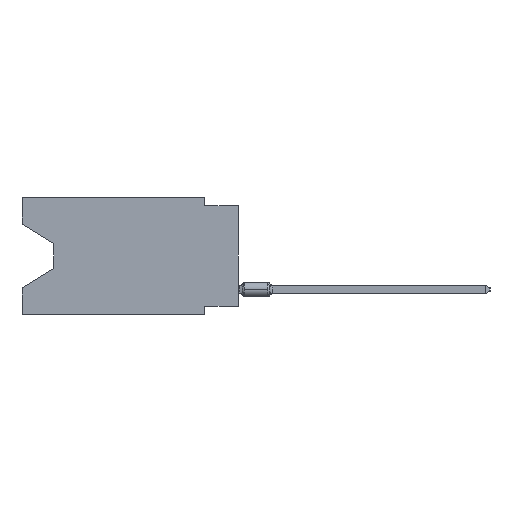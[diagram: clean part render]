
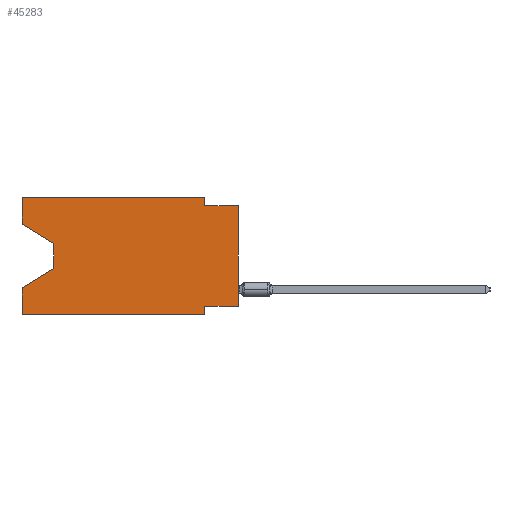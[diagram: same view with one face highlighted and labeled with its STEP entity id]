
A CAD part, left-side view. The second image highlights one B-rep face of the part: STEP entity #45283.
In plain terms, the highlighted planar face has unit normal (-1, 0, 0).
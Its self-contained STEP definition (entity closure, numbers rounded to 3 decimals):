
#516 = EDGE_CURVE ( 'NONE', #14917, #9543, #1992, .T. ) ;
#1327 = CARTESIAN_POINT ( 'NONE',  ( 0., 13.97, -5.385 ) ) ;
#1767 = LINE ( 'NONE', #17411, #11857 ) ;
#1992 = LINE ( 'NONE', #2253, #34191 ) ;
#2253 = CARTESIAN_POINT ( 'NONE',  ( 0., 16.383, -2.038 ) ) ;
#2542 = VECTOR ( 'NONE', #33363, 1000. ) ;
#2892 = VERTEX_POINT ( 'NONE', #22735 ) ;
#2940 = LINE ( 'NONE', #46184, #41017 ) ;
#3522 = CARTESIAN_POINT ( 'NONE',  ( 0., 16.383, 0. ) ) ;
#3793 = DIRECTION ( 'NONE',  ( 1., 0., 0. ) ) ;
#3966 = VECTOR ( 'NONE', #41997, 1000. ) ;
#4473 = VECTOR ( 'NONE', #34867, 1000. ) ;
#5000 = LINE ( 'NONE', #12959, #21048 ) ;
#5082 = CARTESIAN_POINT ( 'NONE',  ( 0., 16.383, 0. ) ) ;
#6580 = CARTESIAN_POINT ( 'NONE',  ( 0., 0., -8.255 ) ) ;
#6715 = LINE ( 'NONE', #37948, #2542 ) ;
#6970 = VECTOR ( 'NONE', #30922, 1000. ) ;
#7168 = ORIENTED_EDGE ( 'NONE', *, *, #42177, .F. ) ;
#8255 = VERTEX_POINT ( 'NONE', #30023 ) ;
#8639 = VERTEX_POINT ( 'NONE', #40820 ) ;
#9111 = DIRECTION ( 'NONE',  ( 0., -1., 0. ) ) ;
#9205 = EDGE_CURVE ( 'NONE', #42547, #8639, #19503, .T. ) ;
#9543 = VERTEX_POINT ( 'NONE', #41468 ) ;
#11857 = VECTOR ( 'NONE', #32268, 1000. ) ;
#12143 = EDGE_CURVE ( 'NONE', #8255, #49991, #5000, .T. ) ;
#12901 = CARTESIAN_POINT ( 'NONE',  ( 0., 0., 0. ) ) ;
#12959 = CARTESIAN_POINT ( 'NONE',  ( 0., 0., -0.635 ) ) ;
#13042 = ORIENTED_EDGE ( 'NONE', *, *, #18100, .F. ) ;
#14010 = EDGE_CURVE ( 'NONE', #20271, #48665, #39620, .T. ) ;
#14073 = CARTESIAN_POINT ( 'NONE',  ( 0., 16.383, -6.852 ) ) ;
#14858 = CARTESIAN_POINT ( 'NONE',  ( 0., 16.383, -8.89 ) ) ;
#14917 = VERTEX_POINT ( 'NONE', #18050 ) ;
#15325 = LINE ( 'NONE', #15568, #6970 ) ;
#15461 = EDGE_CURVE ( 'NONE', #22792, #8639, #39693, .T. ) ;
#15568 = CARTESIAN_POINT ( 'NONE',  ( 0., 13.97, -3.505 ) ) ;
#16507 = PLANE ( 'NONE',  #19033 ) ;
#16711 = CARTESIAN_POINT ( 'NONE',  ( 0., 16.383, 0. ) ) ;
#17411 = CARTESIAN_POINT ( 'NONE',  ( 0., 2.54, 0. ) ) ;
#18050 = CARTESIAN_POINT ( 'NONE',  ( 0., 16.383, -2.038 ) ) ;
#18100 = EDGE_CURVE ( 'NONE', #2892, #8255, #1767, .T. ) ;
#18133 = DIRECTION ( 'NONE',  ( 0., -0.855, -0.519 ) ) ;
#19033 = AXIS2_PLACEMENT_3D ( 'NONE', #3522, #3793, #38588 ) ;
#19503 = LINE ( 'NONE', #42770, #4473 ) ;
#20271 = VERTEX_POINT ( 'NONE', #1327 ) ;
#21048 = VECTOR ( 'NONE', #9111, 1000. ) ;
#21423 = ORIENTED_EDGE ( 'NONE', *, *, #14010, .T. ) ;
#22512 = CARTESIAN_POINT ( 'NONE',  ( 0., 0., -0.635 ) ) ;
#22615 = ORIENTED_EDGE ( 'NONE', *, *, #15461, .F. ) ;
#22735 = CARTESIAN_POINT ( 'NONE',  ( 0., 2.54, 0. ) ) ;
#22792 = VERTEX_POINT ( 'NONE', #42399 ) ;
#22929 = ORIENTED_EDGE ( 'NONE', *, *, #12143, .F. ) ;
#24029 = CARTESIAN_POINT ( 'NONE',  ( 0., 13.97, -5.385 ) ) ;
#24306 = LINE ( 'NONE', #5082, #40575 ) ;
#24942 = EDGE_CURVE ( 'NONE', #29100, #49991, #47685, .T. ) ;
#27446 = CARTESIAN_POINT ( 'NONE',  ( 0., 16.383, 0. ) ) ;
#27990 = DIRECTION ( 'NONE',  ( 0., 0., 1. ) ) ;
#28440 = DIRECTION ( 'NONE',  ( 0., 0., -1. ) ) ;
#29100 = VERTEX_POINT ( 'NONE', #6580 ) ;
#29361 = EDGE_LOOP ( 'NONE', ( #46754, #34235, #21423, #42304, #40164, #22615, #49719, #36845, #22929, #13042, #7168, #47385 ) ) ;
#30023 = CARTESIAN_POINT ( 'NONE',  ( 0., 2.54, -0.635 ) ) ;
#30922 = DIRECTION ( 'NONE',  ( 0., 0., -1. ) ) ;
#31504 = VECTOR ( 'NONE', #34871, 1000. ) ;
#32268 = DIRECTION ( 'NONE',  ( 0., 0., -1. ) ) ;
#33363 = DIRECTION ( 'NONE',  ( 0., 1., 0. ) ) ;
#33942 = EDGE_CURVE ( 'NONE', #29100, #22792, #6715, .T. ) ;
#34191 = VECTOR ( 'NONE', #18133, 1000. ) ;
#34235 = ORIENTED_EDGE ( 'NONE', *, *, #37583, .T. ) ;
#34695 = EDGE_CURVE ( 'NONE', #42547, #48665, #2940, .T. ) ;
#34867 = DIRECTION ( 'NONE',  ( 0., -1., 0. ) ) ;
#34871 = DIRECTION ( 'NONE',  ( 0., -1., 0. ) ) ;
#36845 = ORIENTED_EDGE ( 'NONE', *, *, #24942, .T. ) ;
#37583 = EDGE_CURVE ( 'NONE', #9543, #20271, #15325, .T. ) ;
#37948 = CARTESIAN_POINT ( 'NONE',  ( 0., 0., -8.255 ) ) ;
#38336 = FACE_OUTER_BOUND ( 'NONE', #29361, .T. ) ;
#38588 = DIRECTION ( 'NONE',  ( 0., 0., -1. ) ) ;
#39620 = LINE ( 'NONE', #24029, #3966 ) ;
#39693 = LINE ( 'NONE', #47622, #44975 ) ;
#39892 = DIRECTION ( 'NONE',  ( 0., 0., 1. ) ) ;
#40164 = ORIENTED_EDGE ( 'NONE', *, *, #9205, .T. ) ;
#40575 = VECTOR ( 'NONE', #39892, 1000. ) ;
#40820 = CARTESIAN_POINT ( 'NONE',  ( 0., 2.54, -8.89 ) ) ;
#41017 = VECTOR ( 'NONE', #49275, 1000. ) ;
#41468 = CARTESIAN_POINT ( 'NONE',  ( 0., 13.97, -3.505 ) ) ;
#41997 = DIRECTION ( 'NONE',  ( 0., 0.855, -0.519 ) ) ;
#42177 = EDGE_CURVE ( 'NONE', #49962, #2892, #42529, .T. ) ;
#42304 = ORIENTED_EDGE ( 'NONE', *, *, #34695, .F. ) ;
#42399 = CARTESIAN_POINT ( 'NONE',  ( 0., 2.54, -8.255 ) ) ;
#42529 = LINE ( 'NONE', #27446, #31504 ) ;
#42547 = VERTEX_POINT ( 'NONE', #14858 ) ;
#42733 = EDGE_CURVE ( 'NONE', #14917, #49962, #24306, .T. ) ;
#42770 = CARTESIAN_POINT ( 'NONE',  ( 0., 16.383, -8.89 ) ) ;
#44006 = VECTOR ( 'NONE', #27990, 1000. ) ;
#44975 = VECTOR ( 'NONE', #28440, 1000. ) ;
#45283 = ADVANCED_FACE ( 'NONE', ( #38336 ), #16507, .F. ) ;
#46184 = CARTESIAN_POINT ( 'NONE',  ( 0., 16.383, 0. ) ) ;
#46754 = ORIENTED_EDGE ( 'NONE', *, *, #516, .T. ) ;
#47385 = ORIENTED_EDGE ( 'NONE', *, *, #42733, .F. ) ;
#47622 = CARTESIAN_POINT ( 'NONE',  ( 0., 2.54, -8.89 ) ) ;
#47685 = LINE ( 'NONE', #12901, #44006 ) ;
#48665 = VERTEX_POINT ( 'NONE', #14073 ) ;
#49275 = DIRECTION ( 'NONE',  ( 0., 0., 1. ) ) ;
#49719 = ORIENTED_EDGE ( 'NONE', *, *, #33942, .F. ) ;
#49962 = VERTEX_POINT ( 'NONE', #16711 ) ;
#49991 = VERTEX_POINT ( 'NONE', #22512 ) ;
